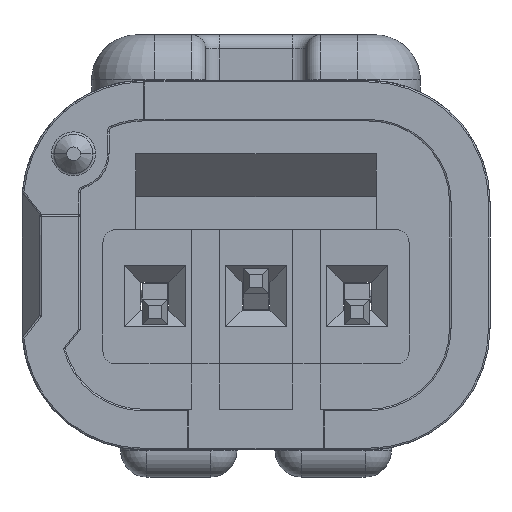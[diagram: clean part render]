
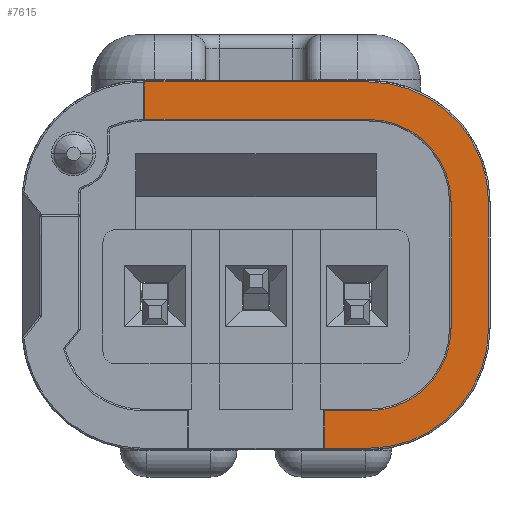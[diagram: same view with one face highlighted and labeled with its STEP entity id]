
A CAD part, front view. The second image highlights one B-rep face of the part: STEP entity #7615.
In plain terms, the highlighted face is planar.
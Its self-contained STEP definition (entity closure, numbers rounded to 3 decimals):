
#244 = EDGE_CURVE ( 'NONE', #9269, #11384, #15634, .T. ) ;
#644 = VERTEX_POINT ( 'NONE', #12698 ) ;
#691 = LINE ( 'NONE', #3836, #17590 ) ;
#780 = DIRECTION ( 'NONE',  ( 0., 0., 1. ) ) ;
#977 = VERTEX_POINT ( 'NONE', #15444 ) ;
#1709 = CARTESIAN_POINT ( 'NONE',  ( 7.55, -1.25, -2.225 ) ) ;
#1723 = EDGE_CURVE ( 'NONE', #11384, #10570, #691, .T. ) ;
#2439 = VECTOR ( 'NONE', #7559, 1000. ) ;
#2605 = CIRCLE ( 'NONE', #13265, 2.37 ) ;
#2768 = DIRECTION ( 'NONE',  ( 1., 0., 0. ) ) ;
#2808 = DIRECTION ( 'NONE',  ( 0., 0., -1. ) ) ;
#2929 = VECTOR ( 'NONE', #9919, 1000. ) ;
#2941 = EDGE_CURVE ( 'NONE', #7789, #5380, #4096, .T. ) ;
#3293 = VERTEX_POINT ( 'NONE', #15798 ) ;
#3663 = VERTEX_POINT ( 'NONE', #15675 ) ;
#3836 = CARTESIAN_POINT ( 'NONE',  ( 7.55, 3.62, 2.225 ) ) ;
#4032 = DIRECTION ( 'NONE',  ( 0., 0., 1. ) ) ;
#4096 = LINE ( 'NONE', #5809, #4154 ) ;
#4154 = VECTOR ( 'NONE', #11421, 1000. ) ;
#4167 = VERTEX_POINT ( 'NONE', #13515 ) ;
#4277 = CARTESIAN_POINT ( 'NONE',  ( 7.55, 1.25, -4.595 ) ) ;
#4296 = FACE_OUTER_BOUND ( 'NONE', #17895, .T. ) ;
#4389 = DIRECTION ( 'NONE',  ( 0., 1., 0. ) ) ;
#4604 = ORIENTED_EDGE ( 'NONE', *, *, #244, .T. ) ;
#4881 = EDGE_CURVE ( 'NONE', #5380, #644, #2605, .T. ) ;
#5103 = ORIENTED_EDGE ( 'NONE', *, *, #8839, .T. ) ;
#5380 = VERTEX_POINT ( 'NONE', #11643 ) ;
#5614 = ORIENTED_EDGE ( 'NONE', *, *, #5820, .T. ) ;
#5649 = CARTESIAN_POINT ( 'NONE',  ( 7.55, 2.85, 2.195 ) ) ;
#5809 = CARTESIAN_POINT ( 'NONE',  ( 7.55, -3.62, -2.225 ) ) ;
#5820 = EDGE_CURVE ( 'NONE', #644, #9269, #13498, .T. ) ;
#6610 = ORIENTED_EDGE ( 'NONE', *, *, #13602, .T. ) ;
#6681 = AXIS2_PLACEMENT_3D ( 'NONE', #15646, #2768, #4389 ) ;
#6868 = LINE ( 'NONE', #18725, #15086 ) ;
#7379 = CARTESIAN_POINT ( 'NONE',  ( 7.55, -1.25, -3.855 ) ) ;
#7408 = AXIS2_PLACEMENT_3D ( 'NONE', #11749, #9833, #14522 ) ;
#7493 = CARTESIAN_POINT ( 'NONE',  ( 7.55, 1.25, -4.595 ) ) ;
#7524 = DIRECTION ( 'NONE',  ( -1., 0., 0. ) ) ;
#7559 = DIRECTION ( 'NONE',  ( 0., -1., 0. ) ) ;
#7615 = ADVANCED_FACE ( 'NONE', ( #4296 ), #18717, .T. ) ;
#7789 = VERTEX_POINT ( 'NONE', #16121 ) ;
#7837 = EDGE_CURVE ( 'NONE', #3293, #977, #18292, .T. ) ;
#8194 = CARTESIAN_POINT ( 'NONE',  ( 7.55, 3.62, -2.225 ) ) ;
#8760 = CIRCLE ( 'NONE', #11205, 1.63 ) ;
#8839 = EDGE_CURVE ( 'NONE', #10570, #13811, #11177, .T. ) ;
#9269 = VERTEX_POINT ( 'NONE', #4277 ) ;
#9313 = EDGE_CURVE ( 'NONE', #4167, #7789, #12944, .T. ) ;
#9833 = DIRECTION ( 'NONE',  ( 1., 0., 0. ) ) ;
#9919 = DIRECTION ( 'NONE',  ( 0., -1., 0. ) ) ;
#9937 = CARTESIAN_POINT ( 'NONE',  ( 7.55, -1.25, -2.225 ) ) ;
#10570 = VERTEX_POINT ( 'NONE', #13118 ) ;
#10758 = DIRECTION ( 'NONE',  ( 0., 0., -1. ) ) ;
#11128 = ORIENTED_EDGE ( 'NONE', *, *, #18752, .T. ) ;
#11177 = LINE ( 'NONE', #5649, #2929 ) ;
#11205 = AXIS2_PLACEMENT_3D ( 'NONE', #15069, #13463, #10758 ) ;
#11384 = VERTEX_POINT ( 'NONE', #8194 ) ;
#11387 = CARTESIAN_POINT ( 'NONE',  ( 7.55, 2.88, -2.225 ) ) ;
#11421 = DIRECTION ( 'NONE',  ( 0., 0., -1. ) ) ;
#11479 = DIRECTION ( 'NONE',  ( 0., 0., -1. ) ) ;
#11609 = ORIENTED_EDGE ( 'NONE', *, *, #17764, .T. ) ;
#11643 = CARTESIAN_POINT ( 'NONE',  ( 7.55, -3.62, -2.225 ) ) ;
#11749 = CARTESIAN_POINT ( 'NONE',  ( 7.55, 1.25, -2.225 ) ) ;
#12066 = DIRECTION ( 'NONE',  ( 0., 1., 0. ) ) ;
#12250 = ORIENTED_EDGE ( 'NONE', *, *, #9313, .T. ) ;
#12698 = CARTESIAN_POINT ( 'NONE',  ( 7.55, -1.25, -4.595 ) ) ;
#12944 = LINE ( 'NONE', #18786, #13910 ) ;
#13118 = CARTESIAN_POINT ( 'NONE',  ( 7.55, 3.62, 2.195 ) ) ;
#13143 = DIRECTION ( 'NONE',  ( 0., -1., 0. ) ) ;
#13190 = ORIENTED_EDGE ( 'NONE', *, *, #4881, .T. ) ;
#13265 = AXIS2_PLACEMENT_3D ( 'NONE', #9937, #15876, #2808 ) ;
#13347 = DIRECTION ( 'NONE',  ( 0., 0., -1. ) ) ;
#13463 = DIRECTION ( 'NONE',  ( -1., 0., 0. ) ) ;
#13498 = LINE ( 'NONE', #7493, #18222 ) ;
#13515 = CARTESIAN_POINT ( 'NONE',  ( 7.55, -2.88, -1.355 ) ) ;
#13602 = EDGE_CURVE ( 'NONE', #977, #4167, #6868, .T. ) ;
#13811 = VERTEX_POINT ( 'NONE', #16512 ) ;
#13910 = VECTOR ( 'NONE', #13143, 1000. ) ;
#14053 = VECTOR ( 'NONE', #11479, 1000. ) ;
#14086 = ORIENTED_EDGE ( 'NONE', *, *, #1723, .T. ) ;
#14384 = ORIENTED_EDGE ( 'NONE', *, *, #16432, .T. ) ;
#14522 = DIRECTION ( 'NONE',  ( 0., 0., -1. ) ) ;
#15069 = CARTESIAN_POINT ( 'NONE',  ( 7.55, 1.25, -2.225 ) ) ;
#15086 = VECTOR ( 'NONE', #4032, 1000. ) ;
#15444 = CARTESIAN_POINT ( 'NONE',  ( 7.55, -2.88, -2.225 ) ) ;
#15634 = CIRCLE ( 'NONE', #7408, 2.37 ) ;
#15646 = CARTESIAN_POINT ( 'NONE',  ( 7.55, -1.25, 2.225 ) ) ;
#15657 = VERTEX_POINT ( 'NONE', #16019 ) ;
#15675 = CARTESIAN_POINT ( 'NONE',  ( 7.55, 2.88, -2.225 ) ) ;
#15798 = CARTESIAN_POINT ( 'NONE',  ( 7.55, -1.25, -3.855 ) ) ;
#15876 = DIRECTION ( 'NONE',  ( 1., 0., 0. ) ) ;
#15981 = ORIENTED_EDGE ( 'NONE', *, *, #2941, .T. ) ;
#15984 = ORIENTED_EDGE ( 'NONE', *, *, #7837, .T. ) ;
#16019 = CARTESIAN_POINT ( 'NONE',  ( 7.55, 1.25, -3.855 ) ) ;
#16121 = CARTESIAN_POINT ( 'NONE',  ( 7.55, -3.62, -1.355 ) ) ;
#16432 = EDGE_CURVE ( 'NONE', #3663, #15657, #8760, .T. ) ;
#16512 = CARTESIAN_POINT ( 'NONE',  ( 7.55, 2.88, 2.195 ) ) ;
#16764 = AXIS2_PLACEMENT_3D ( 'NONE', #1709, #7524, #13347 ) ;
#17035 = LINE ( 'NONE', #11387, #14053 ) ;
#17507 = LINE ( 'NONE', #7379, #2439 ) ;
#17590 = VECTOR ( 'NONE', #780, 1000. ) ;
#17764 = EDGE_CURVE ( 'NONE', #15657, #3293, #17507, .T. ) ;
#17895 = EDGE_LOOP ( 'NONE', ( #12250, #15981, #13190, #5614, #4604, #14086, #5103, #11128, #14384, #11609, #15984, #6610 ) ) ;
#18222 = VECTOR ( 'NONE', #12066, 1000. ) ;
#18292 = CIRCLE ( 'NONE', #16764, 1.63 ) ;
#18717 = PLANE ( 'NONE',  #6681 ) ;
#18725 = CARTESIAN_POINT ( 'NONE',  ( 7.55, -2.88, -1.325 ) ) ;
#18752 = EDGE_CURVE ( 'NONE', #13811, #3663, #17035, .T. ) ;
#18786 = CARTESIAN_POINT ( 'NONE',  ( 7.55, -3.65, -1.355 ) ) ;
